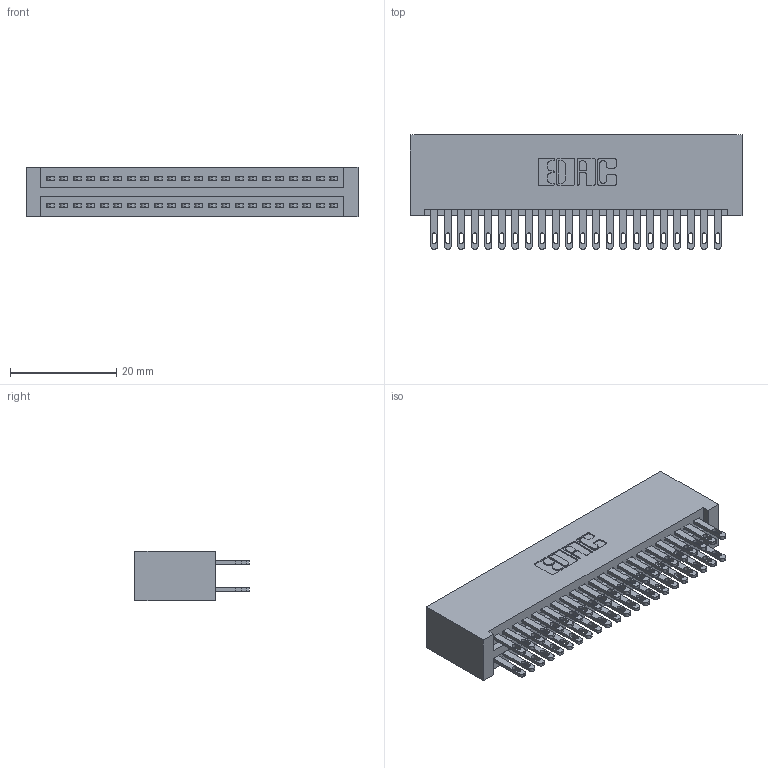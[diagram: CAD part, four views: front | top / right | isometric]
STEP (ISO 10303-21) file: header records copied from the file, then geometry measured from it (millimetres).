
FILE_DESCRIPTION (( 'STEP AP203' ), '1' );
FILE_NAME ('345-044-500-201.STEP', '2018-09-08T07:54:11', ( '' ), ( '' ), 'SwSTEP 2.0', 'SolidWorks 2016', '' );
FILE_SCHEMA (( 'CONFIG_CONTROL_DESIGN' ));
Length unit declared in the file: inch
Products named in the file (3): 345 Part_No Mounting Lugs; 345-292-001_345-293-100; 345-044-500-201
Assembly tree (45 placements, depth 2):
  345-044-500-201
    345 Part_No Mounting Lugs
    345-292-001_345-293-100  x44
Bounding box: 62.48 x 21.51 x 9.4 mm (x, y, z)
Volume: 6634.5 mm3; surface area: 10171.6 mm2
Topology: 45 solids, 45 shells, 2142 faces, 6521 edges, 4346 vertices
Faces by surface type: plane 1264, cylinder 878
Entity records: 19607 total; most frequent: CARTESIAN_POINT 3304, ORIENTED_EDGE 3238, DIRECTION 2935, EDGE_CURVE 1619, LINE 1403, VECTOR 1403, VERTEX_POINT 1078, AXIS2_PLACEMENT_3D 766
